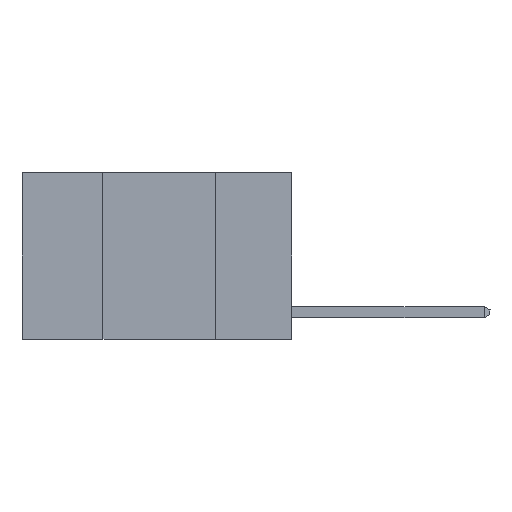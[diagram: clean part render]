
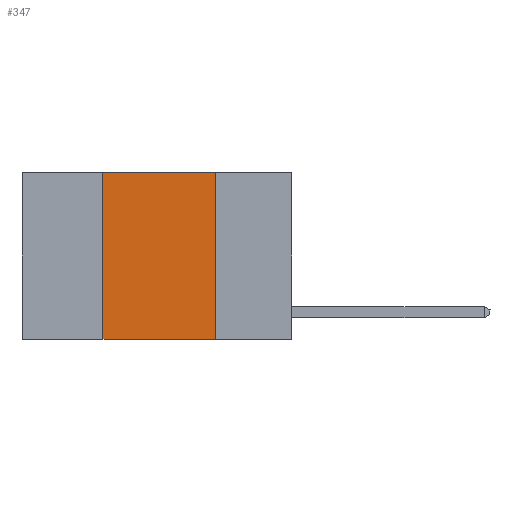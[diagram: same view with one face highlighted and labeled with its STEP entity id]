
A CAD part, left-side view. The second image highlights one B-rep face of the part: STEP entity #347.
In plain terms, the highlighted planar face has unit normal (-1, 0, 0).
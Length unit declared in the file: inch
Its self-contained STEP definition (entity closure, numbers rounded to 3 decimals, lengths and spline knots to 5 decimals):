
#130 = CARTESIAN_POINT ( 'NONE',  ( 0., 0.42, 0. ) ) ;
#200 = DIRECTION ( 'NONE',  ( 0., 0., 1. ) ) ;
#347 = ADVANCED_FACE ( 'NONE', ( #4396 ), #6039, .F. ) ;
#1092 = ORIENTED_EDGE ( 'NONE', *, *, #9340, .F. ) ;
#1360 = DIRECTION ( 'NONE',  ( 0., -1., 0. ) ) ;
#1403 = CARTESIAN_POINT ( 'NONE',  ( 0., 0.42, -0.37 ) ) ;
#1508 = EDGE_CURVE ( 'NONE', #13936, #10560, #9507, .T. ) ;
#3529 = EDGE_LOOP ( 'NONE', ( #12829, #1092, #13154, #10577 ) ) ;
#3768 = CARTESIAN_POINT ( 'NONE',  ( 0., 0.6, -0.37 ) ) ;
#4396 = FACE_OUTER_BOUND ( 'NONE', #3529, .T. ) ;
#4467 = VECTOR ( 'NONE', #200, 39.37008 ) ;
#4752 = VERTEX_POINT ( 'NONE', #1403 ) ;
#4933 = EDGE_CURVE ( 'NONE', #4752, #8510, #13494, .T. ) ;
#4984 = VECTOR ( 'NONE', #10668, 39.37008 ) ;
#5389 = LINE ( 'NONE', #3768, #4984 ) ;
#5726 = DIRECTION ( 'NONE',  ( 0., 0., -1. ) ) ;
#6039 = PLANE ( 'NONE',  #13818 ) ;
#6080 = VECTOR ( 'NONE', #10394, 39.37008 ) ;
#7423 = CARTESIAN_POINT ( 'NONE',  ( 0., 0.17, -0.37 ) ) ;
#8510 = VERTEX_POINT ( 'NONE', #13505 ) ;
#9340 = EDGE_CURVE ( 'NONE', #8510, #13936, #11223, .T. ) ;
#9436 = CARTESIAN_POINT ( 'NONE',  ( 0., 0.6, 0. ) ) ;
#9507 = LINE ( 'NONE', #10254, #6080 ) ;
#10254 = CARTESIAN_POINT ( 'NONE',  ( 0., 0.17, 0. ) ) ;
#10394 = DIRECTION ( 'NONE',  ( 0., 0., -1. ) ) ;
#10560 = VERTEX_POINT ( 'NONE', #7423 ) ;
#10577 = ORIENTED_EDGE ( 'NONE', *, *, #13027, .T. ) ;
#10668 = DIRECTION ( 'NONE',  ( 0., -1., 0. ) ) ;
#11223 = LINE ( 'NONE', #9436, #14410 ) ;
#11490 = DIRECTION ( 'NONE',  ( 1., 0., 0. ) ) ;
#12495 = CARTESIAN_POINT ( 'NONE',  ( 0., 0.6, 0. ) ) ;
#12522 = CARTESIAN_POINT ( 'NONE',  ( 0., 0.17, 0. ) ) ;
#12829 = ORIENTED_EDGE ( 'NONE', *, *, #1508, .F. ) ;
#13027 = EDGE_CURVE ( 'NONE', #4752, #10560, #5389, .T. ) ;
#13154 = ORIENTED_EDGE ( 'NONE', *, *, #4933, .F. ) ;
#13494 = LINE ( 'NONE', #130, #4467 ) ;
#13505 = CARTESIAN_POINT ( 'NONE',  ( 0., 0.42, 0. ) ) ;
#13818 = AXIS2_PLACEMENT_3D ( 'NONE', #12495, #11490, #5726 ) ;
#13936 = VERTEX_POINT ( 'NONE', #12522 ) ;
#14410 = VECTOR ( 'NONE', #1360, 39.37008 ) ;
